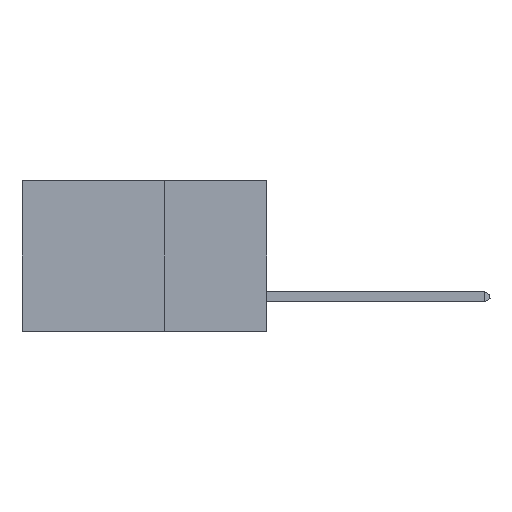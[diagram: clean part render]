
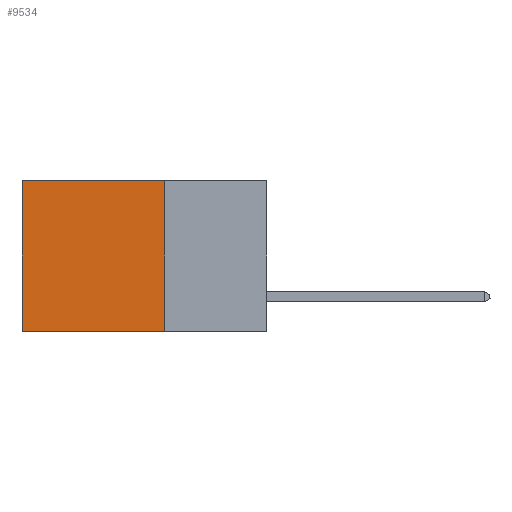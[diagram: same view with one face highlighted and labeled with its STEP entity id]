
A CAD part, left-side view. The second image highlights one B-rep face of the part: STEP entity #9534.
In plain terms, the highlighted planar face has unit normal (-1, 0, 0).
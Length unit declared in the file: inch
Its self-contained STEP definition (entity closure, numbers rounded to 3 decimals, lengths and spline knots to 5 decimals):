
#527 = DIRECTION ( 'NONE',  ( 1., 0., 0. ) ) ;
#1368 = DIRECTION ( 'NONE',  ( 0., 1., 0. ) ) ;
#1906 = VERTEX_POINT ( 'NONE', #19486 ) ;
#2583 = ORIENTED_EDGE ( 'NONE', *, *, #14009, .F. ) ;
#2672 = CARTESIAN_POINT ( 'NONE',  ( 0.2875, 0.25, -0.37 ) ) ;
#3337 = VERTEX_POINT ( 'NONE', #20395 ) ;
#3988 = AXIS2_PLACEMENT_3D ( 'NONE', #20546, #527, #12219 ) ;
#4168 = LINE ( 'NONE', #2672, #10905 ) ;
#5626 = ORIENTED_EDGE ( 'NONE', *, *, #17543, .T. ) ;
#5884 = LINE ( 'NONE', #17688, #17660 ) ;
#6210 = EDGE_CURVE ( 'NONE', #3337, #1906, #4168, .T. ) ;
#6458 = VERTEX_POINT ( 'NONE', #16866 ) ;
#6714 = CARTESIAN_POINT ( 'NONE',  ( 0.2875, 0.25, 0. ) ) ;
#7148 = VECTOR ( 'NONE', #15374, 39.37008 ) ;
#9534 = ADVANCED_FACE ( 'NONE', ( #19602 ), #10531, .F. ) ;
#10531 = PLANE ( 'NONE',  #3988 ) ;
#10731 = VECTOR ( 'NONE', #17860, 39.37008 ) ;
#10905 = VECTOR ( 'NONE', #1368, 39.37008 ) ;
#11307 = CARTESIAN_POINT ( 'NONE',  ( 0.2875, 0.6, 0. ) ) ;
#11758 = LINE ( 'NONE', #12844, #10731 ) ;
#12219 = DIRECTION ( 'NONE',  ( 0., 0., -1. ) ) ;
#12844 = CARTESIAN_POINT ( 'NONE',  ( 0.2875, 0.25, 0. ) ) ;
#13050 = EDGE_LOOP ( 'NONE', ( #5626, #20166, #2583, #14713 ) ) ;
#14009 = EDGE_CURVE ( 'NONE', #6458, #3337, #11758, .T. ) ;
#14713 = ORIENTED_EDGE ( 'NONE', *, *, #18380, .T. ) ;
#15374 = DIRECTION ( 'NONE',  ( 0., 1., 0. ) ) ;
#16866 = CARTESIAN_POINT ( 'NONE',  ( 0.2875, 0.25, 0. ) ) ;
#17104 = LINE ( 'NONE', #6714, #7148 ) ;
#17543 = EDGE_CURVE ( 'NONE', #20290, #1906, #5884, .T. ) ;
#17660 = VECTOR ( 'NONE', #19525, 39.37008 ) ;
#17688 = CARTESIAN_POINT ( 'NONE',  ( 0.2875, 0.6, 0. ) ) ;
#17860 = DIRECTION ( 'NONE',  ( 0., 0., -1. ) ) ;
#18380 = EDGE_CURVE ( 'NONE', #6458, #20290, #17104, .T. ) ;
#19486 = CARTESIAN_POINT ( 'NONE',  ( 0.2875, 0.6, -0.37 ) ) ;
#19525 = DIRECTION ( 'NONE',  ( 0., 0., -1. ) ) ;
#19602 = FACE_OUTER_BOUND ( 'NONE', #13050, .T. ) ;
#20166 = ORIENTED_EDGE ( 'NONE', *, *, #6210, .F. ) ;
#20290 = VERTEX_POINT ( 'NONE', #11307 ) ;
#20395 = CARTESIAN_POINT ( 'NONE',  ( 0.2875, 0.25, -0.37 ) ) ;
#20546 = CARTESIAN_POINT ( 'NONE',  ( 0.2875, 0.25, 0. ) ) ;
